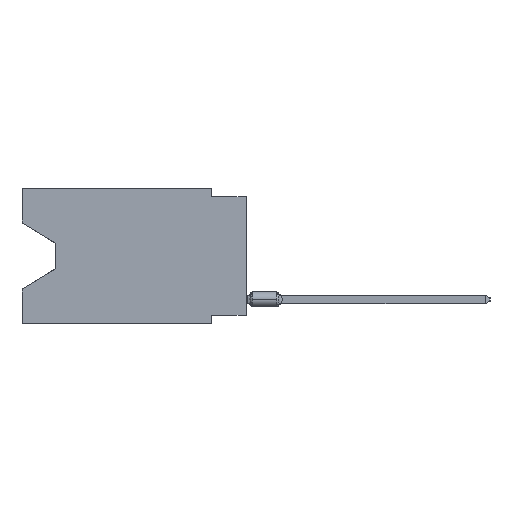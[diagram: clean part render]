
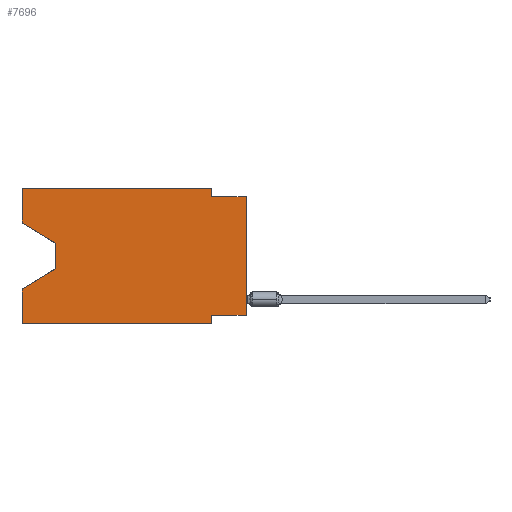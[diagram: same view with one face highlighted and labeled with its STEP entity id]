
A CAD part, left-side view. The second image highlights one B-rep face of the part: STEP entity #7696.
In plain terms, the highlighted planar face has unit normal (-1, 0, 0).
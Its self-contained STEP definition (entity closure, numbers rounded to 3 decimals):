
#535 = CARTESIAN_POINT ( 'NONE',  ( 0., 2.54, -0.635 ) ) ;
#2803 = CARTESIAN_POINT ( 'NONE',  ( 0., 16.383, -7.36 ) ) ;
#3086 = CARTESIAN_POINT ( 'NONE',  ( 0., 2.54, -9.906 ) ) ;
#3795 = LINE ( 'NONE', #74298, #34335 ) ;
#4136 = VERTEX_POINT ( 'NONE', #48266 ) ;
#5150 = EDGE_CURVE ( 'NONE', #33484, #56734, #69471, .T. ) ;
#6668 = DIRECTION ( 'NONE',  ( 0., 0.855, -0.519 ) ) ;
#6979 = CARTESIAN_POINT ( 'NONE',  ( 0., 2.54, -9.271 ) ) ;
#7284 = CARTESIAN_POINT ( 'NONE',  ( 0., 16.383, -2.546 ) ) ;
#7696 = ADVANCED_FACE ( 'NONE', ( #48452 ), #25444, .F. ) ;
#8097 = DIRECTION ( 'NONE',  ( 0., -1., 0. ) ) ;
#8350 = ORIENTED_EDGE ( 'NONE', *, *, #30943, .T. ) ;
#8685 = ORIENTED_EDGE ( 'NONE', *, *, #37435, .T. ) ;
#9283 = EDGE_CURVE ( 'NONE', #22648, #54583, #55622, .T. ) ;
#9860 = EDGE_CURVE ( 'NONE', #54312, #19407, #3795, .T. ) ;
#13383 = LINE ( 'NONE', #36369, #43434 ) ;
#13802 = ORIENTED_EDGE ( 'NONE', *, *, #71134, .T. ) ;
#14538 = AXIS2_PLACEMENT_3D ( 'NONE', #66856, #25067, #54981 ) ;
#17112 = CARTESIAN_POINT ( 'NONE',  ( 0., 0., -9.271 ) ) ;
#18021 = VERTEX_POINT ( 'NONE', #59824 ) ;
#19407 = VERTEX_POINT ( 'NONE', #62119 ) ;
#21942 = ORIENTED_EDGE ( 'NONE', *, *, #26299, .F. ) ;
#22648 = VERTEX_POINT ( 'NONE', #535 ) ;
#24853 = ORIENTED_EDGE ( 'NONE', *, *, #46607, .F. ) ;
#25067 = DIRECTION ( 'NONE',  ( 1., 0., 0. ) ) ;
#25444 = PLANE ( 'NONE',  #14538 ) ;
#25569 = LINE ( 'NONE', #49721, #60351 ) ;
#26299 = EDGE_CURVE ( 'NONE', #56734, #19407, #61355, .T. ) ;
#26709 = VECTOR ( 'NONE', #57471, 1000. ) ;
#28661 = LINE ( 'NONE', #52075, #45775 ) ;
#28686 = LINE ( 'NONE', #73293, #26709 ) ;
#30227 = CARTESIAN_POINT ( 'NONE',  ( 0., 13.97, -5.893 ) ) ;
#30943 = EDGE_CURVE ( 'NONE', #61152, #35345, #71070, .T. ) ;
#30992 = DIRECTION ( 'NONE',  ( 0., -1., 0. ) ) ;
#33178 = LINE ( 'NONE', #49691, #74103 ) ;
#33218 = EDGE_CURVE ( 'NONE', #33484, #54583, #58979, .T. ) ;
#33484 = VERTEX_POINT ( 'NONE', #17112 ) ;
#33973 = ORIENTED_EDGE ( 'NONE', *, *, #9283, .F. ) ;
#34335 = VECTOR ( 'NONE', #50163, 1000. ) ;
#35345 = VERTEX_POINT ( 'NONE', #2803 ) ;
#35539 = DIRECTION ( 'NONE',  ( 0., 0., 1. ) ) ;
#35990 = VECTOR ( 'NONE', #6668, 1000. ) ;
#35999 = CARTESIAN_POINT ( 'NONE',  ( 0., 0., -0.635 ) ) ;
#36158 = CARTESIAN_POINT ( 'NONE',  ( 0., 13.97, -5.893 ) ) ;
#36359 = VECTOR ( 'NONE', #45655, 1000. ) ;
#36369 = CARTESIAN_POINT ( 'NONE',  ( 0., 16.383, 0. ) ) ;
#37435 = EDGE_CURVE ( 'NONE', #18021, #61152, #28686, .T. ) ;
#38488 = ORIENTED_EDGE ( 'NONE', *, *, #9860, .T. ) ;
#39077 = EDGE_LOOP ( 'NONE', ( #13802, #8685, #8350, #46667, #38488, #21942, #46180, #50834, #33973, #24853, #75127, #57134 ) ) ;
#39203 = VECTOR ( 'NONE', #8097, 1000. ) ;
#40317 = CARTESIAN_POINT ( 'NONE',  ( 0., 0., -9.271 ) ) ;
#43434 = VECTOR ( 'NONE', #30992, 1000. ) ;
#45655 = DIRECTION ( 'NONE',  ( 0., -0.855, -0.519 ) ) ;
#45775 = VECTOR ( 'NONE', #35539, 1000. ) ;
#46108 = VECTOR ( 'NONE', #63731, 1000. ) ;
#46180 = ORIENTED_EDGE ( 'NONE', *, *, #5150, .F. ) ;
#46607 = EDGE_CURVE ( 'NONE', #57973, #22648, #25569, .T. ) ;
#46667 = ORIENTED_EDGE ( 'NONE', *, *, #68873, .F. ) ;
#47067 = DIRECTION ( 'NONE',  ( 0., 0., 1. ) ) ;
#47201 = EDGE_CURVE ( 'NONE', #63334, #4136, #28661, .T. ) ;
#48266 = CARTESIAN_POINT ( 'NONE',  ( 0., 16.383, 0. ) ) ;
#48452 = FACE_OUTER_BOUND ( 'NONE', #39077, .T. ) ;
#49691 = CARTESIAN_POINT ( 'NONE',  ( 0., 16.383, 0. ) ) ;
#49721 = CARTESIAN_POINT ( 'NONE',  ( 0., 2.54, 0. ) ) ;
#49859 = CARTESIAN_POINT ( 'NONE',  ( 0., 0., -0.635 ) ) ;
#50078 = CARTESIAN_POINT ( 'NONE',  ( 0., 2.54, 0. ) ) ;
#50163 = DIRECTION ( 'NONE',  ( 0., -1., 0. ) ) ;
#50196 = VECTOR ( 'NONE', #67494, 1000. ) ;
#50834 = ORIENTED_EDGE ( 'NONE', *, *, #33218, .T. ) ;
#52075 = CARTESIAN_POINT ( 'NONE',  ( 0., 16.383, 0. ) ) ;
#54312 = VERTEX_POINT ( 'NONE', #61937 ) ;
#54583 = VERTEX_POINT ( 'NONE', #35999 ) ;
#54981 = DIRECTION ( 'NONE',  ( 0., 0., -1. ) ) ;
#55622 = LINE ( 'NONE', #49859, #39203 ) ;
#55846 = VECTOR ( 'NONE', #47067, 1000. ) ;
#56734 = VERTEX_POINT ( 'NONE', #6979 ) ;
#56812 = CARTESIAN_POINT ( 'NONE',  ( 0., 16.383, -2.546 ) ) ;
#57134 = ORIENTED_EDGE ( 'NONE', *, *, #47201, .F. ) ;
#57471 = DIRECTION ( 'NONE',  ( 0., 0., -1. ) ) ;
#57973 = VERTEX_POINT ( 'NONE', #50078 ) ;
#58979 = LINE ( 'NONE', #65125, #55846 ) ;
#59824 = CARTESIAN_POINT ( 'NONE',  ( 0., 13.97, -4.013 ) ) ;
#60351 = VECTOR ( 'NONE', #73863, 1000. ) ;
#61152 = VERTEX_POINT ( 'NONE', #30227 ) ;
#61355 = LINE ( 'NONE', #3086, #50196 ) ;
#61937 = CARTESIAN_POINT ( 'NONE',  ( 0., 16.383, -9.906 ) ) ;
#62119 = CARTESIAN_POINT ( 'NONE',  ( 0., 2.54, -9.906 ) ) ;
#62576 = LINE ( 'NONE', #56812, #36359 ) ;
#63334 = VERTEX_POINT ( 'NONE', #7284 ) ;
#63731 = DIRECTION ( 'NONE',  ( 0., 1., 0. ) ) ;
#65125 = CARTESIAN_POINT ( 'NONE',  ( 0., 0., 0. ) ) ;
#66856 = CARTESIAN_POINT ( 'NONE',  ( 0., 16.383, 0. ) ) ;
#67494 = DIRECTION ( 'NONE',  ( 0., 0., -1. ) ) ;
#68376 = EDGE_CURVE ( 'NONE', #4136, #57973, #13383, .T. ) ;
#68873 = EDGE_CURVE ( 'NONE', #54312, #35345, #33178, .T. ) ;
#69471 = LINE ( 'NONE', #40317, #46108 ) ;
#71070 = LINE ( 'NONE', #36158, #35990 ) ;
#71134 = EDGE_CURVE ( 'NONE', #63334, #18021, #62576, .T. ) ;
#72687 = DIRECTION ( 'NONE',  ( 0., 0., 1. ) ) ;
#73293 = CARTESIAN_POINT ( 'NONE',  ( 0., 13.97, -4.013 ) ) ;
#73863 = DIRECTION ( 'NONE',  ( 0., 0., -1. ) ) ;
#74103 = VECTOR ( 'NONE', #72687, 1000. ) ;
#74298 = CARTESIAN_POINT ( 'NONE',  ( 0., 16.383, -9.906 ) ) ;
#75127 = ORIENTED_EDGE ( 'NONE', *, *, #68376, .F. ) ;
